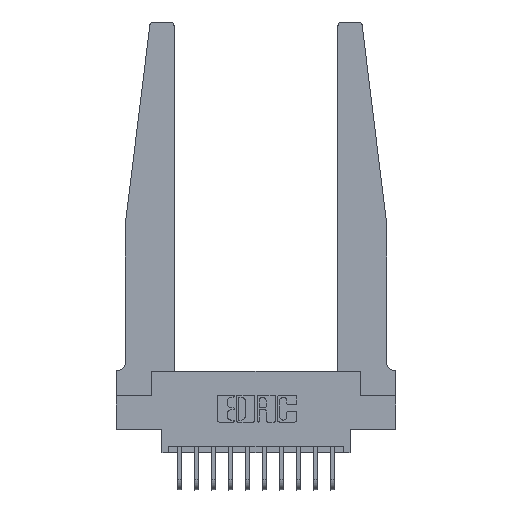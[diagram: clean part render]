
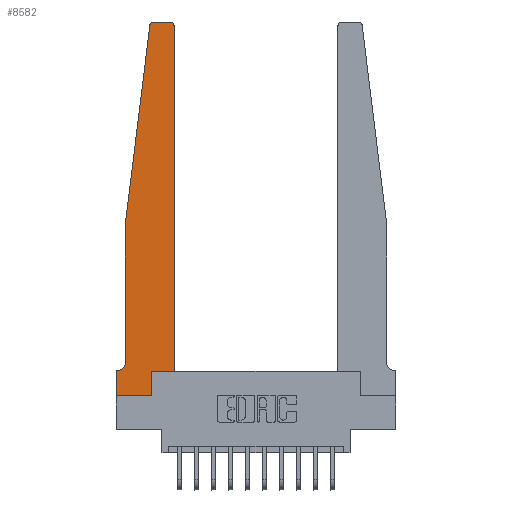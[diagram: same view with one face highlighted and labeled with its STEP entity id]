
A CAD part, top view. The second image highlights one B-rep face of the part: STEP entity #8582.
In plain terms, the highlighted planar face has unit normal (0, 0, 1).
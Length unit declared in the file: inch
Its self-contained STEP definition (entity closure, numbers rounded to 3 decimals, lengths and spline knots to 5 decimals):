
#80 = VERTEX_POINT ( 'NONE', #13435 ) ;
#134 = VERTEX_POINT ( 'NONE', #14884 ) ;
#202 = CARTESIAN_POINT ( 'NONE',  ( 0.24675, 2.72367, 0.37 ) ) ;
#507 = CARTESIAN_POINT ( 'NONE',  ( 0.015, 0.2375, 0.37 ) ) ;
#581 = CIRCLE ( 'NONE', #17411, 0.03 ) ;
#621 = DIRECTION ( 'NONE',  ( -0.122, -0.992, 0. ) ) ;
#691 = CIRCLE ( 'NONE', #3295, 0.05 ) ;
#1066 = VERTEX_POINT ( 'NONE', #9934 ) ;
#1118 = VERTEX_POINT ( 'NONE', #202 ) ;
#1132 = VECTOR ( 'NONE', #621, 39.37008 ) ;
#1510 = ORIENTED_EDGE ( 'NONE', *, *, #13511, .T. ) ;
#1567 = CARTESIAN_POINT ( 'NONE',  ( 0.425, 0.18, 0.37 ) ) ;
#1827 = EDGE_CURVE ( 'NONE', #8211, #2314, #1965, .T. ) ;
#1964 = DIRECTION ( 'NONE',  ( -1., 0., 0. ) ) ;
#1965 = LINE ( 'NONE', #7407, #16380 ) ;
#2027 = CARTESIAN_POINT ( 'NONE',  ( 0.25, 2.75, 0.37 ) ) ;
#2043 = VERTEX_POINT ( 'NONE', #17655 ) ;
#2314 = VERTEX_POINT ( 'NONE', #15762 ) ;
#2447 = EDGE_CURVE ( 'NONE', #16010, #1066, #5112, .T. ) ;
#2725 = VERTEX_POINT ( 'NONE', #14698 ) ;
#3076 = FACE_OUTER_BOUND ( 'NONE', #5614, .T. ) ;
#3090 = LINE ( 'NONE', #16792, #7254 ) ;
#3295 = AXIS2_PLACEMENT_3D ( 'NONE', #507, #6072, #1964 ) ;
#3392 = ORIENTED_EDGE ( 'NONE', *, *, #1827, .T. ) ;
#3407 = VERTEX_POINT ( 'NONE', #8287 ) ;
#3489 = DIRECTION ( 'NONE',  ( 1., 0., 0. ) ) ;
#3854 = CARTESIAN_POINT ( 'NONE',  ( 0.2605, 0.18, 0.37 ) ) ;
#3878 = EDGE_CURVE ( 'NONE', #7424, #80, #10017, .T. ) ;
#3932 = CARTESIAN_POINT ( 'NONE',  ( 0.395, 2.72, 0.37 ) ) ;
#4117 = EDGE_CURVE ( 'NONE', #1066, #1118, #12684, .T. ) ;
#4158 = VECTOR ( 'NONE', #11922, 39.37008 ) ;
#4349 = VECTOR ( 'NONE', #3489, 39.37008 ) ;
#4541 = PLANE ( 'NONE',  #8976 ) ;
#4877 = AXIS2_PLACEMENT_3D ( 'NONE', #16000, #7631, #17174 ) ;
#5098 = LINE ( 'NONE', #10710, #12715 ) ;
#5112 = LINE ( 'NONE', #2027, #4158 ) ;
#5160 = VECTOR ( 'NONE', #5648, 39.37008 ) ;
#5389 = VERTEX_POINT ( 'NONE', #1567 ) ;
#5614 = EDGE_LOOP ( 'NONE', ( #7032, #14774, #17663, #7399, #12266, #1510, #12405, #3392, #11247, #7215, #12808, #11861 ) ) ;
#5648 = DIRECTION ( 'NONE',  ( 0., -1., 0. ) ) ;
#5655 = EDGE_CURVE ( 'NONE', #5389, #2725, #5098, .T. ) ;
#5994 = DIRECTION ( 'NONE',  ( 1., 0., 0. ) ) ;
#6014 = CARTESIAN_POINT ( 'NONE',  ( 0.065, 1.25, 0.37 ) ) ;
#6030 = EDGE_CURVE ( 'NONE', #1118, #7424, #10084, .T. ) ;
#6072 = DIRECTION ( 'NONE',  ( 0., 0., -1. ) ) ;
#6080 = CARTESIAN_POINT ( 'NONE',  ( 0., 0.1875, 0.37 ) ) ;
#6121 = VECTOR ( 'NONE', #16271, 39.37008 ) ;
#6584 = LINE ( 'NONE', #15937, #4349 ) ;
#6820 = DIRECTION ( 'NONE',  ( 0., 1., 0. ) ) ;
#7032 = ORIENTED_EDGE ( 'NONE', *, *, #2447, .T. ) ;
#7215 = ORIENTED_EDGE ( 'NONE', *, *, #9212, .T. ) ;
#7254 = VECTOR ( 'NONE', #12893, 39.37008 ) ;
#7399 = ORIENTED_EDGE ( 'NONE', *, *, #3878, .T. ) ;
#7407 = CARTESIAN_POINT ( 'NONE',  ( 0., 0., 0.37 ) ) ;
#7424 = VERTEX_POINT ( 'NONE', #11326 ) ;
#7436 = CARTESIAN_POINT ( 'NONE',  ( 0., 0., 0.37 ) ) ;
#7462 = EDGE_CURVE ( 'NONE', #2314, #2043, #16307, .T. ) ;
#7583 = DIRECTION ( 'NONE',  ( 1., 0., 0. ) ) ;
#7631 = DIRECTION ( 'NONE',  ( 0., 0., 1. ) ) ;
#8211 = VERTEX_POINT ( 'NONE', #7436 ) ;
#8287 = CARTESIAN_POINT ( 'NONE',  ( 0.015, 0.1875, 0.37 ) ) ;
#8339 = LINE ( 'NONE', #14900, #6121 ) ;
#8582 = ADVANCED_FACE ( 'NONE', ( #3076 ), #4541, .T. ) ;
#8976 = AXIS2_PLACEMENT_3D ( 'NONE', #6080, #10234, #5994 ) ;
#9212 = EDGE_CURVE ( 'NONE', #2043, #5389, #6584, .T. ) ;
#9350 = EDGE_CURVE ( 'NONE', #2725, #16010, #581, .T. ) ;
#9666 = EDGE_CURVE ( 'NONE', #134, #8211, #8339, .T. ) ;
#9934 = CARTESIAN_POINT ( 'NONE',  ( 0.27653, 2.75, 0.37 ) ) ;
#10017 = LINE ( 'NONE', #14188, #5160 ) ;
#10084 = LINE ( 'NONE', #6014, #1132 ) ;
#10234 = DIRECTION ( 'NONE',  ( 0., 0., 1. ) ) ;
#10460 = CARTESIAN_POINT ( 'NONE',  ( 0.395, 2.75, 0.37 ) ) ;
#10497 = DIRECTION ( 'NONE',  ( 0., 1., 0. ) ) ;
#10710 = CARTESIAN_POINT ( 'NONE',  ( 0.425, 0.18, 0.37 ) ) ;
#11247 = ORIENTED_EDGE ( 'NONE', *, *, #7462, .T. ) ;
#11326 = CARTESIAN_POINT ( 'NONE',  ( 0.065, 1.25, 0.37 ) ) ;
#11861 = ORIENTED_EDGE ( 'NONE', *, *, #9350, .T. ) ;
#11922 = DIRECTION ( 'NONE',  ( -1., 0., 0. ) ) ;
#12266 = ORIENTED_EDGE ( 'NONE', *, *, #16798, .T. ) ;
#12405 = ORIENTED_EDGE ( 'NONE', *, *, #9666, .T. ) ;
#12684 = CIRCLE ( 'NONE', #4877, 0.03 ) ;
#12715 = VECTOR ( 'NONE', #6820, 39.37008 ) ;
#12808 = ORIENTED_EDGE ( 'NONE', *, *, #5655, .T. ) ;
#12893 = DIRECTION ( 'NONE',  ( -1., 0., 0. ) ) ;
#13435 = CARTESIAN_POINT ( 'NONE',  ( 0.065, 0.2375, 0.37 ) ) ;
#13511 = EDGE_CURVE ( 'NONE', #3407, #134, #3090, .T. ) ;
#13654 = DIRECTION ( 'NONE',  ( 0., 0., 1. ) ) ;
#14188 = CARTESIAN_POINT ( 'NONE',  ( 0.065, 1.25, 0.37 ) ) ;
#14698 = CARTESIAN_POINT ( 'NONE',  ( 0.425, 2.72, 0.37 ) ) ;
#14774 = ORIENTED_EDGE ( 'NONE', *, *, #4117, .T. ) ;
#14884 = CARTESIAN_POINT ( 'NONE',  ( 0., 0.1875, 0.37 ) ) ;
#14900 = CARTESIAN_POINT ( 'NONE',  ( 0., 0., 0.37 ) ) ;
#15182 = DIRECTION ( 'NONE',  ( 1., 0., 0. ) ) ;
#15762 = CARTESIAN_POINT ( 'NONE',  ( 0.2605, 0., 0.37 ) ) ;
#15937 = CARTESIAN_POINT ( 'NONE',  ( 0.425, 0.18, 0.37 ) ) ;
#16000 = CARTESIAN_POINT ( 'NONE',  ( 0.27653, 2.72, 0.37 ) ) ;
#16010 = VERTEX_POINT ( 'NONE', #10460 ) ;
#16271 = DIRECTION ( 'NONE',  ( 0., -1., 0. ) ) ;
#16307 = LINE ( 'NONE', #3854, #17918 ) ;
#16380 = VECTOR ( 'NONE', #7583, 39.37008 ) ;
#16792 = CARTESIAN_POINT ( 'NONE',  ( 0.065, 0.1875, 0.37 ) ) ;
#16798 = EDGE_CURVE ( 'NONE', #80, #3407, #691, .T. ) ;
#17174 = DIRECTION ( 'NONE',  ( 1., 0., 0. ) ) ;
#17411 = AXIS2_PLACEMENT_3D ( 'NONE', #3932, #13654, #15182 ) ;
#17655 = CARTESIAN_POINT ( 'NONE',  ( 0.2605, 0.18, 0.37 ) ) ;
#17663 = ORIENTED_EDGE ( 'NONE', *, *, #6030, .T. ) ;
#17918 = VECTOR ( 'NONE', #10497, 39.37008 ) ;
